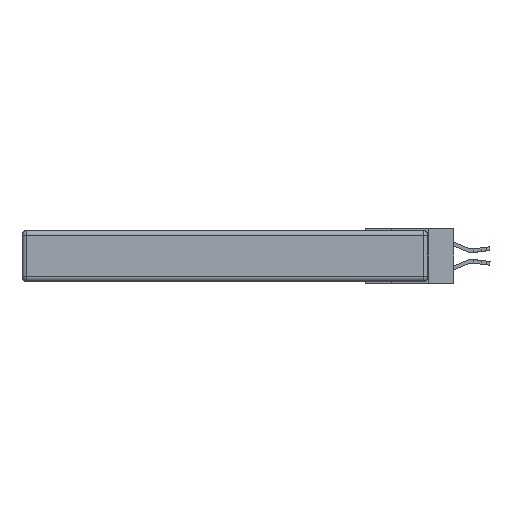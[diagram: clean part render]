
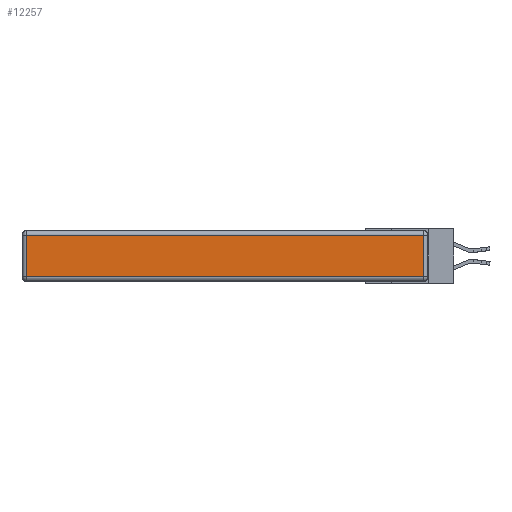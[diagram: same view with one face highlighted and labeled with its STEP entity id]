
A CAD part, left-side view. The second image highlights one B-rep face of the part: STEP entity #12257.
In plain terms, the highlighted planar face has unit normal (-1, 0, 0).
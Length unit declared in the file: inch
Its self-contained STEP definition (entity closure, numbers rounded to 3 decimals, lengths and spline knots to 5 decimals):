
#350 = ORIENTED_EDGE ( 'NONE', *, *, #4669, .T. ) ;
#449 = EDGE_CURVE ( 'NONE', #18650, #16966, #4479, .T. ) ;
#1951 = DIRECTION ( 'NONE',  ( 0., -1., 0. ) ) ;
#2642 = CARTESIAN_POINT ( 'NONE',  ( 0., 0., -0.343 ) ) ;
#2651 = EDGE_LOOP ( 'NONE', ( #5359, #350, #15895, #6419 ) ) ;
#3969 = DIRECTION ( 'NONE',  ( 0., 1., 0. ) ) ;
#4036 = VECTOR ( 'NONE', #1951, 39.37008 ) ;
#4479 = LINE ( 'NONE', #19434, #9038 ) ;
#4669 = EDGE_CURVE ( 'NONE', #12060, #19502, #18344, .T. ) ;
#5359 = ORIENTED_EDGE ( 'NONE', *, *, #15752, .T. ) ;
#6419 = ORIENTED_EDGE ( 'NONE', *, *, #449, .T. ) ;
#7573 = DIRECTION ( 'NONE',  ( 0., 0., -1. ) ) ;
#8408 = CARTESIAN_POINT ( 'NONE',  ( 0., 0.03, -0.313 ) ) ;
#8672 = PLANE ( 'NONE',  #16569 ) ;
#8746 = VECTOR ( 'NONE', #3969, 39.37008 ) ;
#9038 = VECTOR ( 'NONE', #7573, 39.37008 ) ;
#9565 = DIRECTION ( 'NONE',  ( 0., 0., 1. ) ) ;
#10057 = DIRECTION ( 'NONE',  ( -1., 0., 0. ) ) ;
#10121 = DIRECTION ( 'NONE',  ( 0., 0., 1. ) ) ;
#10223 = CARTESIAN_POINT ( 'NONE',  ( 0., 2.72, -0.03 ) ) ;
#10464 = CARTESIAN_POINT ( 'NONE',  ( 0., 0.03, -0.03 ) ) ;
#11798 = LINE ( 'NONE', #13179, #8746 ) ;
#12037 = CARTESIAN_POINT ( 'NONE',  ( 0., 2.72, -0.313 ) ) ;
#12060 = VERTEX_POINT ( 'NONE', #8408 ) ;
#12257 = ADVANCED_FACE ( 'NONE', ( #15547 ), #8672, .T. ) ;
#12623 = LINE ( 'NONE', #18569, #4036 ) ;
#13179 = CARTESIAN_POINT ( 'NONE',  ( 0., 2.75, -0.03 ) ) ;
#15547 = FACE_OUTER_BOUND ( 'NONE', #2651, .T. ) ;
#15752 = EDGE_CURVE ( 'NONE', #16966, #12060, #12623, .T. ) ;
#15895 = ORIENTED_EDGE ( 'NONE', *, *, #18561, .T. ) ;
#16569 = AXIS2_PLACEMENT_3D ( 'NONE', #2642, #10057, #10121 ) ;
#16966 = VERTEX_POINT ( 'NONE', #12037 ) ;
#17178 = CARTESIAN_POINT ( 'NONE',  ( 0., 0.03, -0.343 ) ) ;
#17873 = VECTOR ( 'NONE', #9565, 39.37008 ) ;
#18344 = LINE ( 'NONE', #17178, #17873 ) ;
#18561 = EDGE_CURVE ( 'NONE', #19502, #18650, #11798, .T. ) ;
#18569 = CARTESIAN_POINT ( 'NONE',  ( 0., 0., -0.313 ) ) ;
#18650 = VERTEX_POINT ( 'NONE', #10223 ) ;
#19434 = CARTESIAN_POINT ( 'NONE',  ( 0., 2.72, -0.343 ) ) ;
#19502 = VERTEX_POINT ( 'NONE', #10464 ) ;
